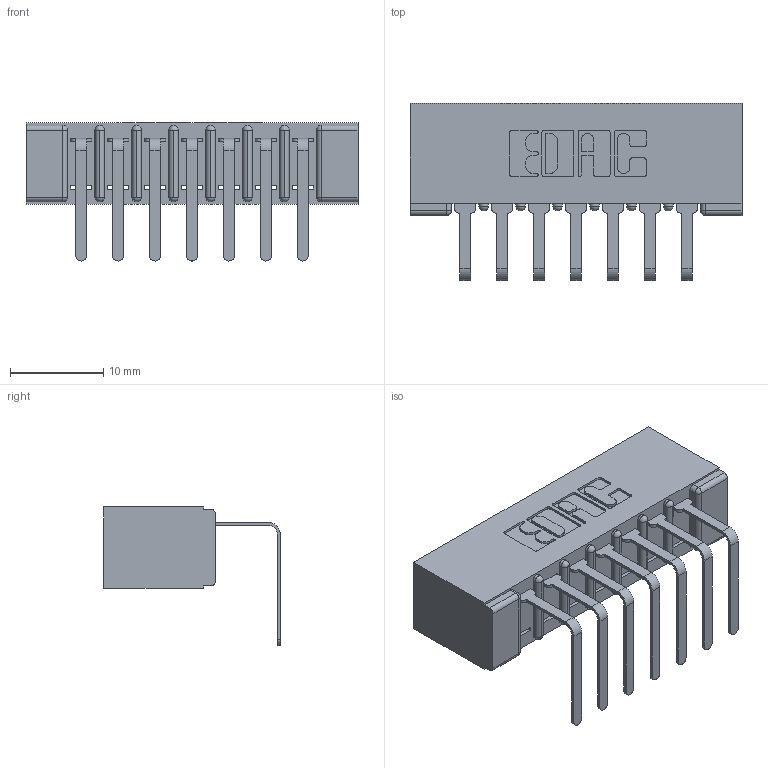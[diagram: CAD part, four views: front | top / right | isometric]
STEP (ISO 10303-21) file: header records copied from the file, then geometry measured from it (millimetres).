
FILE_DESCRIPTION (( 'STEP AP203' ), '1' );
FILE_NAME ('307-007-558-101.STEP', '2019-09-04T11:53:14', ( '' ), ( '' ), 'SwSTEP 2.0', 'SolidWorks 2016', '' );
FILE_SCHEMA (( 'CONFIG_CONTROL_DESIGN' ));
Length unit declared in the file: inch
Products named in the file (3): 307-290-001_558 - 2 (Single); 307 Part_No Mounting Lugs; 307-007-558-101
Assembly tree (8 placements, depth 2):
  307-007-558-101
    307 Part_No Mounting Lugs
    307-290-001_558 - 2 (Single)  x7
Bounding box: 35.61 x 18.96 x 14.81 mm (x, y, z)
Volume: 2516.1 mm3; surface area: 3841.6 mm2
Topology: 8 solids, 8 shells, 538 faces, 1517 edges, 978 vertices
Faces by surface type: plane 339, cylinder 183, sphere 16
Entity records: 10142 total; most frequent: CARTESIAN_POINT 1696, ORIENTED_EDGE 1682, DIRECTION 1669, EDGE_CURVE 841, LINE 631, VECTOR 631, VERTEX_POINT 546, AXIS2_PLACEMENT_3D 519
